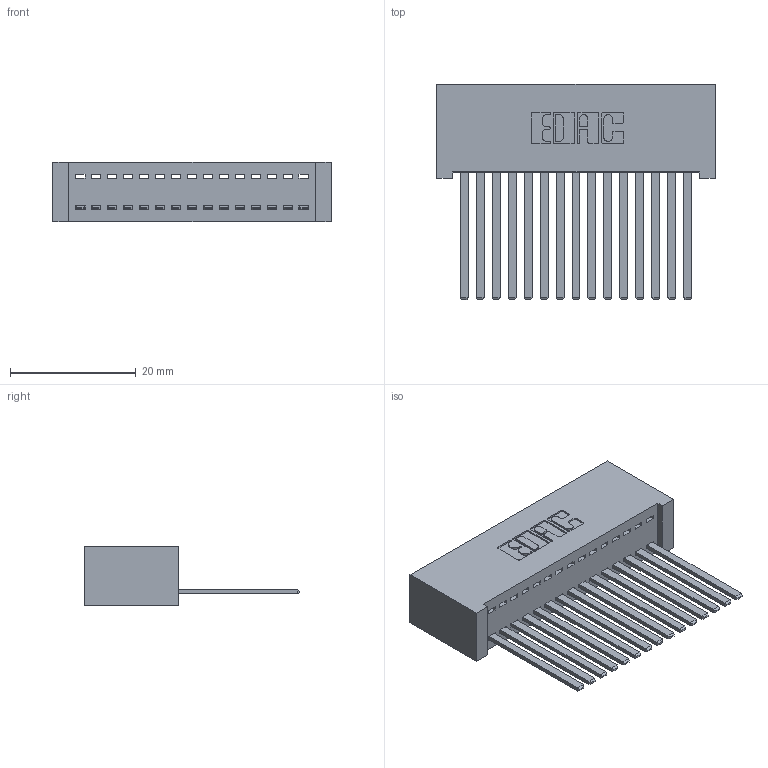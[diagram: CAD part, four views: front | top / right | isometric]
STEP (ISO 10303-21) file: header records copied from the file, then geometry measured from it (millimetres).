
FILE_DESCRIPTION (( 'STEP AP203' ), '1' );
FILE_NAME ('342-015-544-101.STEP', '2019-10-01T18:27:19', ( '' ), ( '' ), 'SwSTEP 2.0', 'SolidWorks 2016', '' );
FILE_SCHEMA (( 'CONFIG_CONTROL_DESIGN' ));
Length unit declared in the file: inch
Products named in the file (3): 342-015-544-101; 342 Part_Lugless; 345-292-001_345-293-144
Assembly tree (16 placements, depth 2):
  342-015-544-101
    342 Part_Lugless
    345-292-001_345-293-144  x15
Bounding box: 44.35 x 34.3 x 9.4 mm (x, y, z)
Volume: 4371.7 mm3; surface area: 6733.2 mm2
Topology: 16 solids, 16 shells, 882 faces, 2645 edges, 1742 vertices
Faces by surface type: plane 632, cylinder 250
Entity records: 12069 total; most frequent: CARTESIAN_POINT 2091, ORIENTED_EDGE 2042, DIRECTION 1807, EDGE_CURVE 1021, LINE 905, VECTOR 905, VERTEX_POINT 678, AXIS2_PLACEMENT_3D 451
